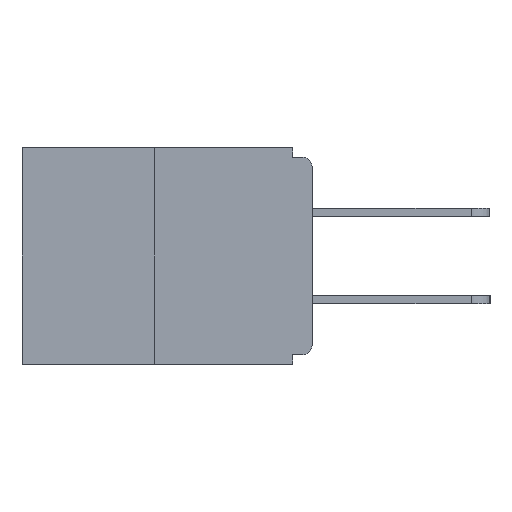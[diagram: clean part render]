
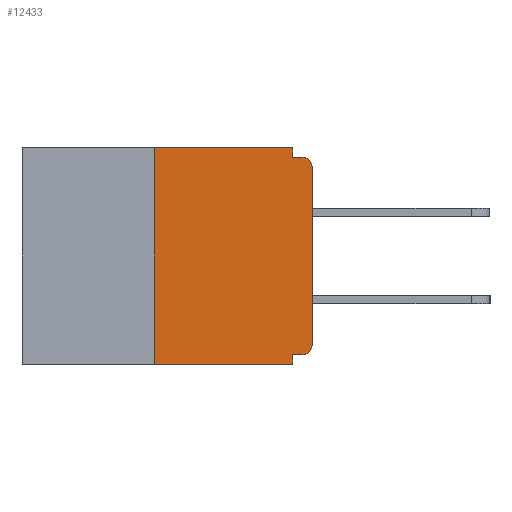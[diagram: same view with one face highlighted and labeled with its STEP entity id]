
A CAD part, left-side view. The second image highlights one B-rep face of the part: STEP entity #12433.
In plain terms, the highlighted planar face has unit normal (-1, 0, 0).
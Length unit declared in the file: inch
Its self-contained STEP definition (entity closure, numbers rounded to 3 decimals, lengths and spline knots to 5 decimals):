
#103 = EDGE_CURVE ( 'NONE', #6389, #7170, #6213, .T. ) ;
#539 = CARTESIAN_POINT ( 'NONE',  ( 0., 0.25, -0.343 ) ) ;
#676 = VECTOR ( 'NONE', #7518, 39.37008 ) ;
#894 = DIRECTION ( 'NONE',  ( 0., 0., -1. ) ) ;
#984 = PLANE ( 'NONE',  #13736 ) ;
#1161 = FACE_OUTER_BOUND ( 'NONE', #1495, .T. ) ;
#1344 = EDGE_CURVE ( 'NONE', #13401, #9167, #1422, .T. ) ;
#1422 = LINE ( 'NONE', #2059, #12823 ) ;
#1495 = EDGE_LOOP ( 'NONE', ( #2072, #10751, #12581, #13062, #5091, #14900, #13117, #13631, #11168, #2432 ) ) ;
#2059 = CARTESIAN_POINT ( 'NONE',  ( 0., 0., -0.328 ) ) ;
#2072 = ORIENTED_EDGE ( 'NONE', *, *, #103, .F. ) ;
#2432 = ORIENTED_EDGE ( 'NONE', *, *, #8699, .F. ) ;
#2495 = LINE ( 'NONE', #2518, #9098 ) ;
#2518 = CARTESIAN_POINT ( 'NONE',  ( 0., 0., -0.015 ) ) ;
#2525 = CARTESIAN_POINT ( 'NONE',  ( 0., 0.25, 0. ) ) ;
#3336 = DIRECTION ( 'NONE',  ( 0., 0., -1. ) ) ;
#4486 = DIRECTION ( 'NONE',  ( 0., 0., -1. ) ) ;
#4573 = AXIS2_PLACEMENT_3D ( 'NONE', #5653, #6674, #4486 ) ;
#4811 = DIRECTION ( 'NONE',  ( 0., -1., 0. ) ) ;
#4958 = DIRECTION ( 'NONE',  ( 0., -1., 0. ) ) ;
#5091 = ORIENTED_EDGE ( 'NONE', *, *, #1344, .F. ) ;
#5587 = VERTEX_POINT ( 'NONE', #12784 ) ;
#5653 = CARTESIAN_POINT ( 'NONE',  ( 0., 0.015, -0.03 ) ) ;
#5707 = DIRECTION ( 'NONE',  ( 0., 0., -1. ) ) ;
#6046 = EDGE_CURVE ( 'NONE', #12890, #5587, #2495, .T. ) ;
#6213 = LINE ( 'NONE', #6435, #13233 ) ;
#6389 = VERTEX_POINT ( 'NONE', #7304 ) ;
#6435 = CARTESIAN_POINT ( 'NONE',  ( 0., 0.46, 0. ) ) ;
#6674 = DIRECTION ( 'NONE',  ( -1., 0., 0. ) ) ;
#7170 = VERTEX_POINT ( 'NONE', #7704 ) ;
#7269 = LINE ( 'NONE', #7711, #8548 ) ;
#7304 = CARTESIAN_POINT ( 'NONE',  ( 0., 0.25, 0. ) ) ;
#7416 = VERTEX_POINT ( 'NONE', #11748 ) ;
#7518 = DIRECTION ( 'NONE',  ( 0., 0., 1. ) ) ;
#7704 = CARTESIAN_POINT ( 'NONE',  ( 0., 0.031, 0. ) ) ;
#7711 = CARTESIAN_POINT ( 'NONE',  ( 0., 0.031, 0. ) ) ;
#7883 = VERTEX_POINT ( 'NONE', #539 ) ;
#8190 = EDGE_CURVE ( 'NONE', #9167, #14460, #14024, .T. ) ;
#8401 = DIRECTION ( 'NONE',  ( 0., 0., 1. ) ) ;
#8548 = VECTOR ( 'NONE', #10175, 39.37008 ) ;
#8659 = CARTESIAN_POINT ( 'NONE',  ( 0., 0.015, -0.328 ) ) ;
#8660 = CARTESIAN_POINT ( 'NONE',  ( 0., 0., 0. ) ) ;
#8699 = EDGE_CURVE ( 'NONE', #7170, #12890, #7269, .T. ) ;
#9098 = VECTOR ( 'NONE', #4958, 39.37008 ) ;
#9167 = VERTEX_POINT ( 'NONE', #14370 ) ;
#9337 = VECTOR ( 'NONE', #8401, 39.37008 ) ;
#9403 = CARTESIAN_POINT ( 'NONE',  ( 0., 0.46, -0.343 ) ) ;
#9666 = CIRCLE ( 'NONE', #4573, 0.015 ) ;
#9947 = DIRECTION ( 'NONE',  ( 0., -1., 0. ) ) ;
#10175 = DIRECTION ( 'NONE',  ( 0., 0., -1. ) ) ;
#10180 = EDGE_CURVE ( 'NONE', #7416, #5587, #9666, .T. ) ;
#10282 = CARTESIAN_POINT ( 'NONE',  ( 0., 0.46, 0. ) ) ;
#10720 = VECTOR ( 'NONE', #5707, 39.37008 ) ;
#10721 = CIRCLE ( 'NONE', #12268, 0.015 ) ;
#10751 = ORIENTED_EDGE ( 'NONE', *, *, #14343, .F. ) ;
#11091 = LINE ( 'NONE', #9403, #12950 ) ;
#11168 = ORIENTED_EDGE ( 'NONE', *, *, #6046, .F. ) ;
#11454 = DIRECTION ( 'NONE',  ( 0., 1., 0. ) ) ;
#11521 = LINE ( 'NONE', #8660, #676 ) ;
#11748 = CARTESIAN_POINT ( 'NONE',  ( 0., 0., -0.03 ) ) ;
#11813 = EDGE_CURVE ( 'NONE', #13401, #12448, #10721, .T. ) ;
#11932 = EDGE_CURVE ( 'NONE', #7883, #14460, #11091, .T. ) ;
#12268 = AXIS2_PLACEMENT_3D ( 'NONE', #13854, #12601, #894 ) ;
#12433 = ADVANCED_FACE ( 'NONE', ( #1161 ), #984, .F. ) ;
#12448 = VERTEX_POINT ( 'NONE', #15162 ) ;
#12470 = LINE ( 'NONE', #2525, #9337 ) ;
#12581 = ORIENTED_EDGE ( 'NONE', *, *, #11932, .T. ) ;
#12601 = DIRECTION ( 'NONE',  ( -1., 0., 0. ) ) ;
#12778 = CARTESIAN_POINT ( 'NONE',  ( 0., 0.031, -0.343 ) ) ;
#12784 = CARTESIAN_POINT ( 'NONE',  ( 0., 0.015, -0.015 ) ) ;
#12823 = VECTOR ( 'NONE', #11454, 39.37008 ) ;
#12890 = VERTEX_POINT ( 'NONE', #14544 ) ;
#12950 = VECTOR ( 'NONE', #4811, 39.37008 ) ;
#13062 = ORIENTED_EDGE ( 'NONE', *, *, #8190, .F. ) ;
#13117 = ORIENTED_EDGE ( 'NONE', *, *, #14722, .T. ) ;
#13233 = VECTOR ( 'NONE', #9947, 39.37008 ) ;
#13401 = VERTEX_POINT ( 'NONE', #8659 ) ;
#13631 = ORIENTED_EDGE ( 'NONE', *, *, #10180, .T. ) ;
#13736 = AXIS2_PLACEMENT_3D ( 'NONE', #10282, #15064, #3336 ) ;
#13854 = CARTESIAN_POINT ( 'NONE',  ( 0., 0.015, -0.313 ) ) ;
#13995 = CARTESIAN_POINT ( 'NONE',  ( 0., 0.031, -0.343 ) ) ;
#14024 = LINE ( 'NONE', #12778, #10720 ) ;
#14343 = EDGE_CURVE ( 'NONE', #7883, #6389, #12470, .T. ) ;
#14370 = CARTESIAN_POINT ( 'NONE',  ( 0., 0.031, -0.328 ) ) ;
#14460 = VERTEX_POINT ( 'NONE', #13995 ) ;
#14544 = CARTESIAN_POINT ( 'NONE',  ( 0., 0.031, -0.015 ) ) ;
#14722 = EDGE_CURVE ( 'NONE', #12448, #7416, #11521, .T. ) ;
#14900 = ORIENTED_EDGE ( 'NONE', *, *, #11813, .T. ) ;
#15064 = DIRECTION ( 'NONE',  ( 1., 0., 0. ) ) ;
#15162 = CARTESIAN_POINT ( 'NONE',  ( 0., 0., -0.313 ) ) ;
